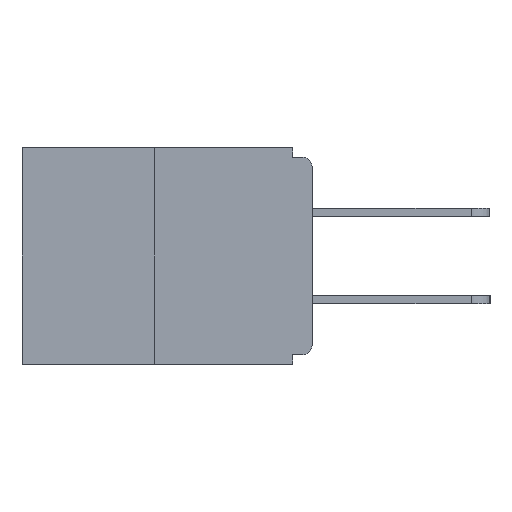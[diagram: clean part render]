
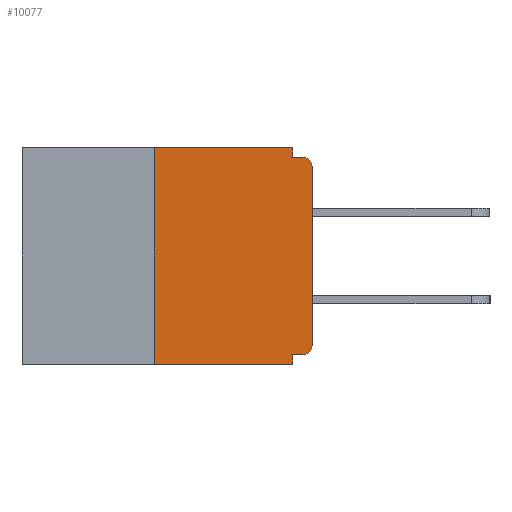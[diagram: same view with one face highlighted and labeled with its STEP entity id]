
A CAD part, left-side view. The second image highlights one B-rep face of the part: STEP entity #10077.
In plain terms, the highlighted planar face has unit normal (-1, 0, 0).
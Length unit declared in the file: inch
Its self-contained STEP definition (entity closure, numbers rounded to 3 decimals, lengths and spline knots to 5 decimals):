
#181 = CARTESIAN_POINT ( 'NONE',  ( 0., 0.46, -0.343 ) ) ;
#265 = DIRECTION ( 'NONE',  ( 0., 0., -1. ) ) ;
#346 = VERTEX_POINT ( 'NONE', #7081 ) ;
#365 = CARTESIAN_POINT ( 'NONE',  ( 0., 0.46, 0. ) ) ;
#476 = PLANE ( 'NONE',  #14125 ) ;
#900 = DIRECTION ( 'NONE',  ( 0., 0., 1. ) ) ;
#908 = ORIENTED_EDGE ( 'NONE', *, *, #1097, .F. ) ;
#1015 = VERTEX_POINT ( 'NONE', #1789 ) ;
#1030 = CIRCLE ( 'NONE', #9566, 0.015 ) ;
#1097 = EDGE_CURVE ( 'NONE', #13349, #2435, #4701, .T. ) ;
#1315 = VECTOR ( 'NONE', #12313, 39.37008 ) ;
#1413 = CARTESIAN_POINT ( 'NONE',  ( 0., 0.031, 0. ) ) ;
#1789 = CARTESIAN_POINT ( 'NONE',  ( 0., 0.015, -0.328 ) ) ;
#1809 = CARTESIAN_POINT ( 'NONE',  ( 0., 0., -0.328 ) ) ;
#2079 = LINE ( 'NONE', #5471, #7485 ) ;
#2165 = EDGE_CURVE ( 'NONE', #11059, #11451, #2449, .T. ) ;
#2262 = ORIENTED_EDGE ( 'NONE', *, *, #5257, .F. ) ;
#2343 = DIRECTION ( 'NONE',  ( 0., 0., -1. ) ) ;
#2435 = VERTEX_POINT ( 'NONE', #14715 ) ;
#2449 = LINE ( 'NONE', #181, #2821 ) ;
#2508 = EDGE_CURVE ( 'NONE', #11059, #6469, #4257, .T. ) ;
#2821 = VECTOR ( 'NONE', #13107, 39.37008 ) ;
#3784 = VECTOR ( 'NONE', #13591, 39.37008 ) ;
#3993 = ORIENTED_EDGE ( 'NONE', *, *, #2165, .T. ) ;
#4257 = LINE ( 'NONE', #6479, #8604 ) ;
#4324 = VECTOR ( 'NONE', #12619, 39.37008 ) ;
#4701 = LINE ( 'NONE', #13443, #5053 ) ;
#4718 = VERTEX_POINT ( 'NONE', #7580 ) ;
#4742 = EDGE_CURVE ( 'NONE', #2435, #4718, #9981, .T. ) ;
#4819 = DIRECTION ( 'NONE',  ( -1., 0., 0. ) ) ;
#5053 = VECTOR ( 'NONE', #6521, 39.37008 ) ;
#5257 = EDGE_CURVE ( 'NONE', #6469, #13349, #13354, .T. ) ;
#5465 = DIRECTION ( 'NONE',  ( 0., 0., -1. ) ) ;
#5471 = CARTESIAN_POINT ( 'NONE',  ( 0., 0.031, -0.343 ) ) ;
#5619 = LINE ( 'NONE', #1809, #1315 ) ;
#5667 = DIRECTION ( 'NONE',  ( 0., 0., -1. ) ) ;
#6390 = AXIS2_PLACEMENT_3D ( 'NONE', #7778, #13446, #5465 ) ;
#6469 = VERTEX_POINT ( 'NONE', #12660 ) ;
#6479 = CARTESIAN_POINT ( 'NONE',  ( 0., 0.25, 0. ) ) ;
#6521 = DIRECTION ( 'NONE',  ( 0., 0., -1. ) ) ;
#7081 = CARTESIAN_POINT ( 'NONE',  ( 0., 0., -0.313 ) ) ;
#7178 = DIRECTION ( 'NONE',  ( 1., 0., 0. ) ) ;
#7485 = VECTOR ( 'NONE', #5667, 39.37008 ) ;
#7566 = EDGE_CURVE ( 'NONE', #12225, #4718, #1030, .T. ) ;
#7580 = CARTESIAN_POINT ( 'NONE',  ( 0., 0.015, -0.015 ) ) ;
#7778 = CARTESIAN_POINT ( 'NONE',  ( 0., 0.015, -0.313 ) ) ;
#8029 = EDGE_CURVE ( 'NONE', #12334, #11451, #2079, .T. ) ;
#8538 = FACE_OUTER_BOUND ( 'NONE', #13265, .T. ) ;
#8546 = CARTESIAN_POINT ( 'NONE',  ( 0., 0.031, -0.343 ) ) ;
#8551 = ORIENTED_EDGE ( 'NONE', *, *, #4742, .F. ) ;
#8604 = VECTOR ( 'NONE', #900, 39.37008 ) ;
#8866 = CARTESIAN_POINT ( 'NONE',  ( 0., 0.25, -0.343 ) ) ;
#8890 = ORIENTED_EDGE ( 'NONE', *, *, #12811, .T. ) ;
#9218 = VECTOR ( 'NONE', #9912, 39.37008 ) ;
#9235 = CARTESIAN_POINT ( 'NONE',  ( 0., 0.46, 0. ) ) ;
#9445 = CARTESIAN_POINT ( 'NONE',  ( 0., 0.015, -0.03 ) ) ;
#9566 = AXIS2_PLACEMENT_3D ( 'NONE', #9445, #4819, #2343 ) ;
#9912 = DIRECTION ( 'NONE',  ( 0., -1., 0. ) ) ;
#9981 = LINE ( 'NONE', #13401, #9218 ) ;
#10077 = ADVANCED_FACE ( 'NONE', ( #8538 ), #476, .F. ) ;
#10126 = CARTESIAN_POINT ( 'NONE',  ( 0., 0., -0.03 ) ) ;
#10217 = CARTESIAN_POINT ( 'NONE',  ( 0., 0.031, -0.328 ) ) ;
#10790 = ORIENTED_EDGE ( 'NONE', *, *, #7566, .T. ) ;
#11059 = VERTEX_POINT ( 'NONE', #8866 ) ;
#11146 = ORIENTED_EDGE ( 'NONE', *, *, #8029, .F. ) ;
#11451 = VERTEX_POINT ( 'NONE', #8546 ) ;
#12222 = EDGE_CURVE ( 'NONE', #1015, #12334, #5619, .T. ) ;
#12225 = VERTEX_POINT ( 'NONE', #10126 ) ;
#12313 = DIRECTION ( 'NONE',  ( 0., 1., 0. ) ) ;
#12334 = VERTEX_POINT ( 'NONE', #10217 ) ;
#12619 = DIRECTION ( 'NONE',  ( 0., -1., 0. ) ) ;
#12660 = CARTESIAN_POINT ( 'NONE',  ( 0., 0.25, 0. ) ) ;
#12811 = EDGE_CURVE ( 'NONE', #346, #12225, #13553, .T. ) ;
#12879 = EDGE_CURVE ( 'NONE', #1015, #346, #13197, .T. ) ;
#13107 = DIRECTION ( 'NONE',  ( 0., -1., 0. ) ) ;
#13197 = CIRCLE ( 'NONE', #6390, 0.015 ) ;
#13265 = EDGE_LOOP ( 'NONE', ( #2262, #13459, #3993, #11146, #13968, #14345, #8890, #10790, #8551, #908 ) ) ;
#13349 = VERTEX_POINT ( 'NONE', #1413 ) ;
#13354 = LINE ( 'NONE', #9235, #4324 ) ;
#13401 = CARTESIAN_POINT ( 'NONE',  ( 0., 0., -0.015 ) ) ;
#13443 = CARTESIAN_POINT ( 'NONE',  ( 0., 0.031, 0. ) ) ;
#13446 = DIRECTION ( 'NONE',  ( -1., 0., 0. ) ) ;
#13459 = ORIENTED_EDGE ( 'NONE', *, *, #2508, .F. ) ;
#13544 = CARTESIAN_POINT ( 'NONE',  ( 0., 0., 0. ) ) ;
#13553 = LINE ( 'NONE', #13544, #3784 ) ;
#13591 = DIRECTION ( 'NONE',  ( 0., 0., 1. ) ) ;
#13968 = ORIENTED_EDGE ( 'NONE', *, *, #12222, .F. ) ;
#14125 = AXIS2_PLACEMENT_3D ( 'NONE', #365, #7178, #265 ) ;
#14345 = ORIENTED_EDGE ( 'NONE', *, *, #12879, .T. ) ;
#14715 = CARTESIAN_POINT ( 'NONE',  ( 0., 0.031, -0.015 ) ) ;
